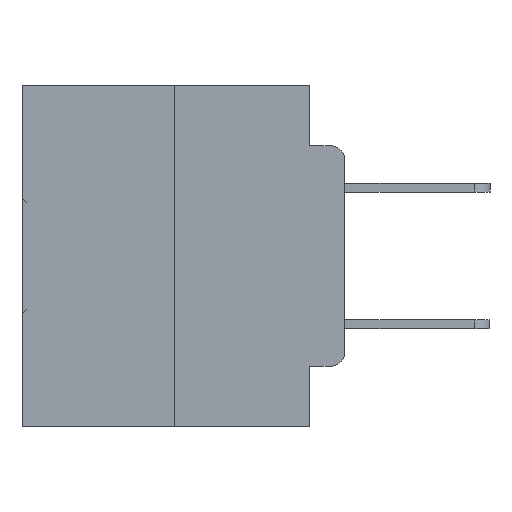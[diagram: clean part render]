
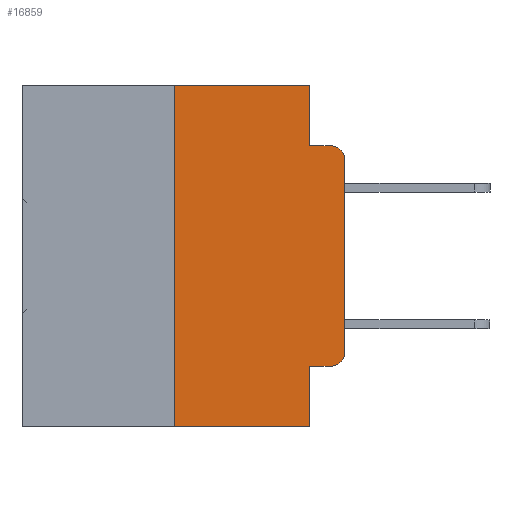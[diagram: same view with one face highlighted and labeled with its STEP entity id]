
A CAD part, left-side view. The second image highlights one B-rep face of the part: STEP entity #16859.
In plain terms, the highlighted planar face has unit normal (-1, 0, 0).
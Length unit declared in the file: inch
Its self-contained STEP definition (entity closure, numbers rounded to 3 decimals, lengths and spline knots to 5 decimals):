
#489 = LINE ( 'NONE', #13274, #7620 ) ;
#854 = CARTESIAN_POINT ( 'NONE',  ( 0., 0.051, -0.4115 ) ) ;
#1133 = EDGE_CURVE ( 'NONE', #14164, #20746, #489, .T. ) ;
#2808 = CARTESIAN_POINT ( 'NONE',  ( 0., 0.051, 0. ) ) ;
#3793 = VERTEX_POINT ( 'NONE', #6534 ) ;
#4061 = VERTEX_POINT ( 'NONE', #10332 ) ;
#4600 = LINE ( 'NONE', #26756, #10830 ) ;
#5484 = DIRECTION ( 'NONE',  ( 1., 0., 0. ) ) ;
#5499 = DIRECTION ( 'NONE',  ( 0., 0., -1. ) ) ;
#6309 = ORIENTED_EDGE ( 'NONE', *, *, #32526, .T. ) ;
#6326 = ORIENTED_EDGE ( 'NONE', *, *, #32575, .T. ) ;
#6354 = VECTOR ( 'NONE', #5499, 39.37008 ) ;
#6504 = DIRECTION ( 'NONE',  ( -1., 0., 0. ) ) ;
#6534 = CARTESIAN_POINT ( 'NONE',  ( 0., 0.02, -0.4115 ) ) ;
#6791 = ORIENTED_EDGE ( 'NONE', *, *, #10280, .F. ) ;
#7468 = CARTESIAN_POINT ( 'NONE',  ( 0., 0., -0.1085 ) ) ;
#7620 = VECTOR ( 'NONE', #13164, 39.37008 ) ;
#7786 = EDGE_CURVE ( 'NONE', #20746, #11487, #24888, .T. ) ;
#8496 = CARTESIAN_POINT ( 'NONE',  ( 0., 0.25, 0. ) ) ;
#8662 = ORIENTED_EDGE ( 'NONE', *, *, #33677, .F. ) ;
#8835 = VERTEX_POINT ( 'NONE', #21133 ) ;
#9303 = VERTEX_POINT ( 'NONE', #15528 ) ;
#9560 = AXIS2_PLACEMENT_3D ( 'NONE', #11827, #30283, #14453 ) ;
#10280 = EDGE_CURVE ( 'NONE', #9303, #11487, #17255, .T. ) ;
#10332 = CARTESIAN_POINT ( 'NONE',  ( 0., 0.051, -0.4115 ) ) ;
#10830 = VECTOR ( 'NONE', #24060, 39.37008 ) ;
#11110 = ORIENTED_EDGE ( 'NONE', *, *, #21028, .F. ) ;
#11487 = VERTEX_POINT ( 'NONE', #27990 ) ;
#11547 = VERTEX_POINT ( 'NONE', #23012 ) ;
#11584 = DIRECTION ( 'NONE',  ( 0., -1., 0. ) ) ;
#11827 = CARTESIAN_POINT ( 'NONE',  ( 0., 0.02, -0.1085 ) ) ;
#13164 = DIRECTION ( 'NONE',  ( 0., 0., 1. ) ) ;
#13274 = CARTESIAN_POINT ( 'NONE',  ( 0., 0., 0. ) ) ;
#13586 = VECTOR ( 'NONE', #19065, 39.37008 ) ;
#13730 = LINE ( 'NONE', #8496, #33923 ) ;
#13804 = DIRECTION ( 'NONE',  ( 0., 0., 1. ) ) ;
#14164 = VERTEX_POINT ( 'NONE', #28205 ) ;
#14239 = LINE ( 'NONE', #854, #27509 ) ;
#14453 = DIRECTION ( 'NONE',  ( 0., 0., -1. ) ) ;
#15226 = LINE ( 'NONE', #29567, #13586 ) ;
#15528 = CARTESIAN_POINT ( 'NONE',  ( 0., 0.051, -0.0885 ) ) ;
#16248 = EDGE_CURVE ( 'NONE', #8835, #29092, #15226, .T. ) ;
#16410 = VECTOR ( 'NONE', #18099, 39.37008 ) ;
#16859 = ADVANCED_FACE ( 'NONE', ( #30475 ), #21375, .F. ) ;
#17255 = LINE ( 'NONE', #33860, #16410 ) ;
#17515 = ORIENTED_EDGE ( 'NONE', *, *, #16248, .T. ) ;
#18099 = DIRECTION ( 'NONE',  ( 0., -1., 0. ) ) ;
#18555 = ORIENTED_EDGE ( 'NONE', *, *, #7786, .T. ) ;
#18842 = CARTESIAN_POINT ( 'NONE',  ( 0., 0.473, 0. ) ) ;
#19065 = DIRECTION ( 'NONE',  ( 0., -1., 0. ) ) ;
#19251 = CARTESIAN_POINT ( 'NONE',  ( 0., 0.051, -0.5 ) ) ;
#20110 = ORIENTED_EDGE ( 'NONE', *, *, #1133, .T. ) ;
#20597 = AXIS2_PLACEMENT_3D ( 'NONE', #31847, #5484, #24008 ) ;
#20746 = VERTEX_POINT ( 'NONE', #7468 ) ;
#21028 = EDGE_CURVE ( 'NONE', #8835, #11547, #13730, .T. ) ;
#21133 = CARTESIAN_POINT ( 'NONE',  ( 0., 0.25, -0.5 ) ) ;
#21375 = PLANE ( 'NONE',  #20597 ) ;
#22097 = EDGE_CURVE ( 'NONE', #24044, #9303, #4600, .T. ) ;
#22109 = EDGE_CURVE ( 'NONE', #11547, #24044, #32709, .T. ) ;
#22353 = CARTESIAN_POINT ( 'NONE',  ( 0., 0.02, -0.3915 ) ) ;
#23012 = CARTESIAN_POINT ( 'NONE',  ( 0., 0.25, 0. ) ) ;
#23225 = EDGE_LOOP ( 'NONE', ( #20110, #18555, #6791, #34152, #27473, #11110, #17515, #8662, #6309, #6326 ) ) ;
#24008 = DIRECTION ( 'NONE',  ( 0., 0., -1. ) ) ;
#24044 = VERTEX_POINT ( 'NONE', #27534 ) ;
#24060 = DIRECTION ( 'NONE',  ( 0., 0., -1. ) ) ;
#24888 = CIRCLE ( 'NONE', #9560, 0.02 ) ;
#25008 = DIRECTION ( 'NONE',  ( 0., 0., -1. ) ) ;
#26756 = CARTESIAN_POINT ( 'NONE',  ( 0., 0.051, 0. ) ) ;
#27465 = LINE ( 'NONE', #2808, #6354 ) ;
#27473 = ORIENTED_EDGE ( 'NONE', *, *, #22109, .F. ) ;
#27509 = VECTOR ( 'NONE', #11584, 39.37008 ) ;
#27534 = CARTESIAN_POINT ( 'NONE',  ( 0., 0.051, 0. ) ) ;
#27990 = CARTESIAN_POINT ( 'NONE',  ( 0., 0.02, -0.0885 ) ) ;
#28205 = CARTESIAN_POINT ( 'NONE',  ( 0., 0., -0.3915 ) ) ;
#28442 = AXIS2_PLACEMENT_3D ( 'NONE', #22353, #6504, #25008 ) ;
#29092 = VERTEX_POINT ( 'NONE', #19251 ) ;
#29354 = DIRECTION ( 'NONE',  ( 0., -1., 0. ) ) ;
#29567 = CARTESIAN_POINT ( 'NONE',  ( 0., 0.473, -0.5 ) ) ;
#30283 = DIRECTION ( 'NONE',  ( -1., 0., 0. ) ) ;
#30475 = FACE_OUTER_BOUND ( 'NONE', #23225, .T. ) ;
#31058 = VECTOR ( 'NONE', #29354, 39.37008 ) ;
#31847 = CARTESIAN_POINT ( 'NONE',  ( 0., 0.473, 0. ) ) ;
#32526 = EDGE_CURVE ( 'NONE', #4061, #3793, #14239, .T. ) ;
#32575 = EDGE_CURVE ( 'NONE', #3793, #14164, #33631, .T. ) ;
#32709 = LINE ( 'NONE', #18842, #31058 ) ;
#33631 = CIRCLE ( 'NONE', #28442, 0.02 ) ;
#33677 = EDGE_CURVE ( 'NONE', #4061, #29092, #27465, .T. ) ;
#33860 = CARTESIAN_POINT ( 'NONE',  ( 0., 0.051, -0.0885 ) ) ;
#33923 = VECTOR ( 'NONE', #13804, 39.37008 ) ;
#34152 = ORIENTED_EDGE ( 'NONE', *, *, #22097, .F. ) ;
